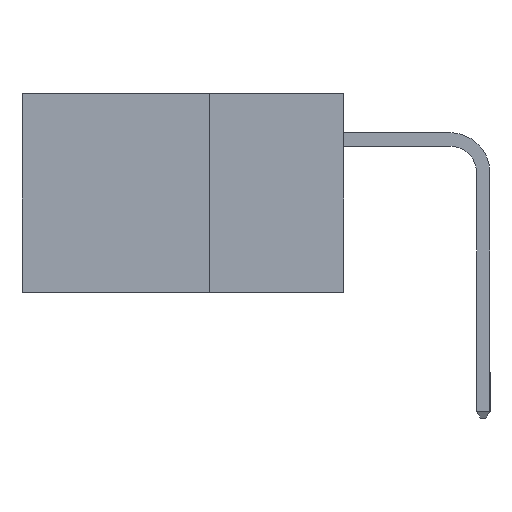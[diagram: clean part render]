
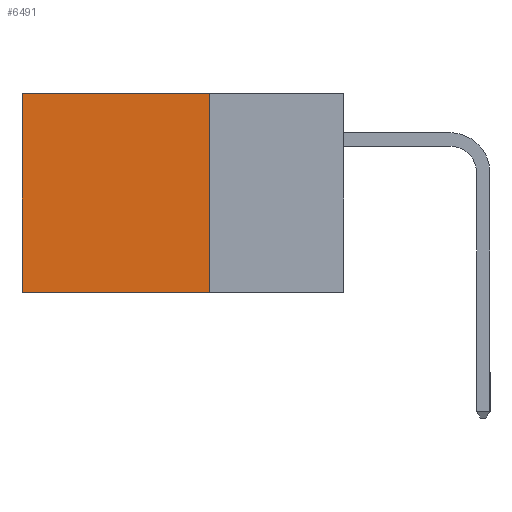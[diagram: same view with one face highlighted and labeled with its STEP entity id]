
A CAD part, left-side view. The second image highlights one B-rep face of the part: STEP entity #6491.
In plain terms, the highlighted planar face has unit normal (-1, 0, 0).
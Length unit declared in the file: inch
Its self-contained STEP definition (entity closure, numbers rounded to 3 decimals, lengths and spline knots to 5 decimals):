
#195 = VERTEX_POINT ( 'NONE', #4883 ) ;
#242 = EDGE_CURVE ( 'NONE', #6351, #5395, #4144, .T. ) ;
#271 = DIRECTION ( 'NONE',  ( 0., 0., -1. ) ) ;
#387 = ORIENTED_EDGE ( 'NONE', *, *, #6921, .F. ) ;
#466 = LINE ( 'NONE', #6568, #8692 ) ;
#550 = EDGE_LOOP ( 'NONE', ( #2441, #8747, #387, #7853 ) ) ;
#1370 = VECTOR ( 'NONE', #271, 39.37008 ) ;
#2385 = PLANE ( 'NONE',  #3230 ) ;
#2441 = ORIENTED_EDGE ( 'NONE', *, *, #7492, .T. ) ;
#2993 = LINE ( 'NONE', #6293, #1370 ) ;
#3105 = VECTOR ( 'NONE', #8025, 39.37008 ) ;
#3230 = AXIS2_PLACEMENT_3D ( 'NONE', #6044, #5362, #5829 ) ;
#3739 = CARTESIAN_POINT ( 'NONE',  ( 0.2615, 0.6, -0.37 ) ) ;
#3779 = DIRECTION ( 'NONE',  ( 0., 1., 0. ) ) ;
#4128 = CARTESIAN_POINT ( 'NONE',  ( 0.2615, 0.25, -0.37 ) ) ;
#4129 = CARTESIAN_POINT ( 'NONE',  ( 0.2615, 0.6, 0. ) ) ;
#4144 = LINE ( 'NONE', #5601, #7284 ) ;
#4883 = CARTESIAN_POINT ( 'NONE',  ( 0.2615, 0.6, -0.37 ) ) ;
#5354 = DIRECTION ( 'NONE',  ( 0., 1., 0. ) ) ;
#5362 = DIRECTION ( 'NONE',  ( 1., 0., 0. ) ) ;
#5395 = VERTEX_POINT ( 'NONE', #4129 ) ;
#5601 = CARTESIAN_POINT ( 'NONE',  ( 0.2615, 0.25, 0. ) ) ;
#5642 = EDGE_CURVE ( 'NONE', #8326, #195, #466, .T. ) ;
#5824 = LINE ( 'NONE', #3739, #3105 ) ;
#5829 = DIRECTION ( 'NONE',  ( 0., 0., -1. ) ) ;
#6044 = CARTESIAN_POINT ( 'NONE',  ( 0.2615, 0.25, -0.37 ) ) ;
#6293 = CARTESIAN_POINT ( 'NONE',  ( 0.2615, 0.25, -0.37 ) ) ;
#6351 = VERTEX_POINT ( 'NONE', #8522 ) ;
#6491 = ADVANCED_FACE ( 'NONE', ( #7855 ), #2385, .F. ) ;
#6568 = CARTESIAN_POINT ( 'NONE',  ( 0.2615, 0.25, -0.37 ) ) ;
#6921 = EDGE_CURVE ( 'NONE', #6351, #8326, #2993, .T. ) ;
#7284 = VECTOR ( 'NONE', #3779, 39.37008 ) ;
#7492 = EDGE_CURVE ( 'NONE', #5395, #195, #5824, .T. ) ;
#7853 = ORIENTED_EDGE ( 'NONE', *, *, #242, .T. ) ;
#7855 = FACE_OUTER_BOUND ( 'NONE', #550, .T. ) ;
#8025 = DIRECTION ( 'NONE',  ( 0., 0., -1. ) ) ;
#8326 = VERTEX_POINT ( 'NONE', #4128 ) ;
#8522 = CARTESIAN_POINT ( 'NONE',  ( 0.2615, 0.25, 0. ) ) ;
#8692 = VECTOR ( 'NONE', #5354, 39.37008 ) ;
#8747 = ORIENTED_EDGE ( 'NONE', *, *, #5642, .F. ) ;
